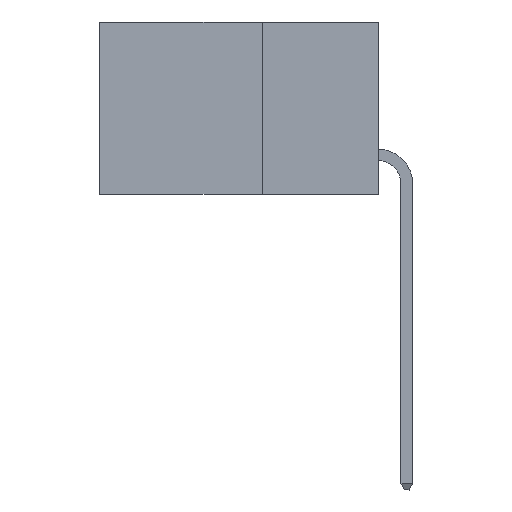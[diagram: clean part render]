
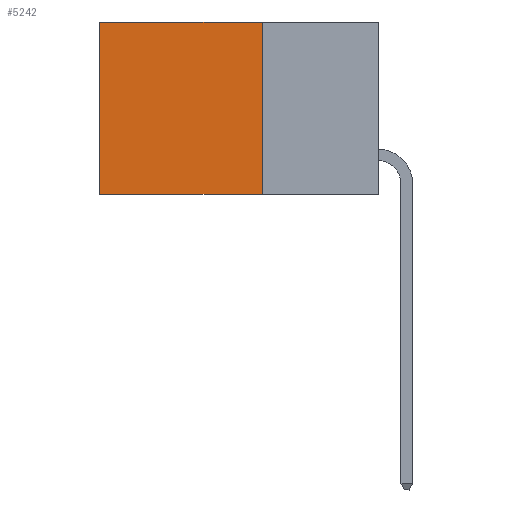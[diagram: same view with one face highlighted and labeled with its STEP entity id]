
A CAD part, left-side view. The second image highlights one B-rep face of the part: STEP entity #5242.
In plain terms, the highlighted planar face has unit normal (-1, 0, 0).
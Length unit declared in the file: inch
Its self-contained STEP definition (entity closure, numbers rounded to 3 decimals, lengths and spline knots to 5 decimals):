
#53 = VERTEX_POINT ( 'NONE', #7735 ) ;
#317 = DIRECTION ( 'NONE',  ( 0., 0., -1. ) ) ;
#529 = AXIS2_PLACEMENT_3D ( 'NONE', #4174, #4917, #2581 ) ;
#852 = DIRECTION ( 'NONE',  ( 0., 1., 0. ) ) ;
#1642 = VERTEX_POINT ( 'NONE', #7165 ) ;
#2022 = VERTEX_POINT ( 'NONE', #8965 ) ;
#2377 = ORIENTED_EDGE ( 'NONE', *, *, #2566, .T. ) ;
#2566 = EDGE_CURVE ( 'NONE', #53, #2022, #8483, .T. ) ;
#2581 = DIRECTION ( 'NONE',  ( 0., 0., -1. ) ) ;
#3155 = VECTOR ( 'NONE', #8419, 39.37008 ) ;
#3401 = VECTOR ( 'NONE', #852, 39.37008 ) ;
#3511 = EDGE_CURVE ( 'NONE', #53, #1642, #4550, .T. ) ;
#3954 = CARTESIAN_POINT ( 'NONE',  ( 0.2615, 0.25, 0. ) ) ;
#4062 = LINE ( 'NONE', #6943, #4240 ) ;
#4125 = EDGE_LOOP ( 'NONE', ( #4397, #5191, #7827, #2377 ) ) ;
#4174 = CARTESIAN_POINT ( 'NONE',  ( 0.2615, 0.25, -0.37 ) ) ;
#4240 = VECTOR ( 'NONE', #317, 39.37008 ) ;
#4397 = ORIENTED_EDGE ( 'NONE', *, *, #6625, .T. ) ;
#4550 = LINE ( 'NONE', #4708, #3155 ) ;
#4674 = DIRECTION ( 'NONE',  ( 0., 1., 0. ) ) ;
#4708 = CARTESIAN_POINT ( 'NONE',  ( 0.2615, 0.25, -0.37 ) ) ;
#4804 = PLANE ( 'NONE',  #529 ) ;
#4917 = DIRECTION ( 'NONE',  ( 1., 0., 0. ) ) ;
#5191 = ORIENTED_EDGE ( 'NONE', *, *, #9284, .F. ) ;
#5242 = ADVANCED_FACE ( 'NONE', ( #7054 ), #4804, .F. ) ;
#5388 = LINE ( 'NONE', #7637, #3401 ) ;
#6625 = EDGE_CURVE ( 'NONE', #2022, #7855, #4062, .T. ) ;
#6756 = VECTOR ( 'NONE', #4674, 39.37008 ) ;
#6943 = CARTESIAN_POINT ( 'NONE',  ( 0.2615, 0.6, -0.37 ) ) ;
#7054 = FACE_OUTER_BOUND ( 'NONE', #4125, .T. ) ;
#7165 = CARTESIAN_POINT ( 'NONE',  ( 0.2615, 0.25, -0.37 ) ) ;
#7637 = CARTESIAN_POINT ( 'NONE',  ( 0.2615, 0.25, -0.37 ) ) ;
#7735 = CARTESIAN_POINT ( 'NONE',  ( 0.2615, 0.25, 0. ) ) ;
#7827 = ORIENTED_EDGE ( 'NONE', *, *, #3511, .F. ) ;
#7855 = VERTEX_POINT ( 'NONE', #8759 ) ;
#8419 = DIRECTION ( 'NONE',  ( 0., 0., -1. ) ) ;
#8483 = LINE ( 'NONE', #3954, #6756 ) ;
#8759 = CARTESIAN_POINT ( 'NONE',  ( 0.2615, 0.6, -0.37 ) ) ;
#8965 = CARTESIAN_POINT ( 'NONE',  ( 0.2615, 0.6, 0. ) ) ;
#9284 = EDGE_CURVE ( 'NONE', #1642, #7855, #5388, .T. ) ;
